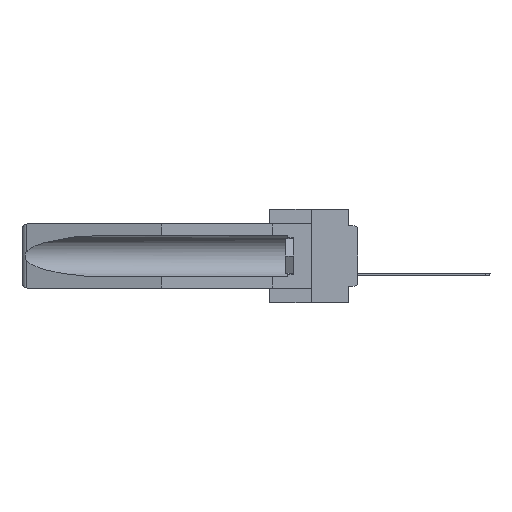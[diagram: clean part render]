
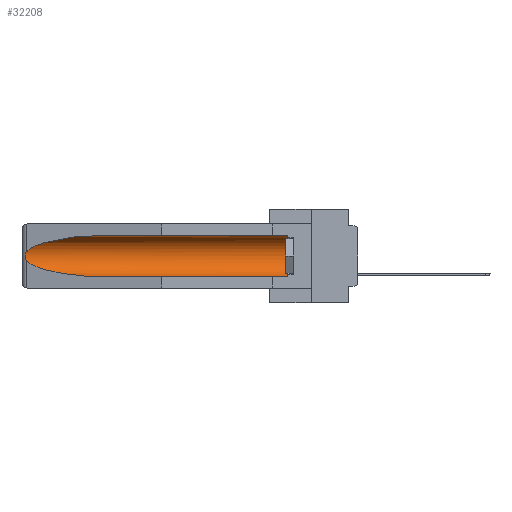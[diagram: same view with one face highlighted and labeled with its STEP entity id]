
A CAD part, left-side view. The second image highlights one B-rep face of the part: STEP entity #32208.
In plain terms, the highlighted cylindrical face has radius 2.857 mm (diameter 5.715 mm), a partial arc.
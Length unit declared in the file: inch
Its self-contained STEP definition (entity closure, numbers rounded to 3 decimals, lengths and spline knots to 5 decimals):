
#1415 = LINE ( 'NONE', #34284, #30825 ) ;
#1539 = VERTEX_POINT ( 'NONE', #34513 ) ;
#1839 = ORIENTED_EDGE ( 'NONE', *, *, #25517, .T. ) ;
#2169 = ORIENTED_EDGE ( 'NONE', *, *, #26123, .T. ) ;
#2974 = ORIENTED_EDGE ( 'NONE', *, *, #4304, .T. ) ;
#4304 = EDGE_CURVE ( 'NONE', #13439, #25281, #10258, .T. ) ;
#6087 = DIRECTION ( 'NONE',  ( 0., 0., 1. ) ) ;
#6419 = DIRECTION ( 'NONE',  ( 0., 1., 0. ) ) ;
#6476 = EDGE_LOOP ( 'NONE', ( #1839, #2169, #2974, #25697, #29636, #35950 ) ) ;
#7685 = CARTESIAN_POINT ( 'NONE',  ( 0.2675, 1.53308, -0.17534 ) ) ;
#7814 = CARTESIAN_POINT ( 'NONE',  ( 0.26655, 1.53094, -0.18657 ) ) ;
#7979 = EDGE_CURVE ( 'NONE', #1539, #15425, #1415, .T. ) ;
#8011 = CARTESIAN_POINT ( 'NONE',  ( 0.21114, 1.30732, -0.059 ) ) ;
#8209 = B_SPLINE_CURVE_WITH_KNOTS ( 'NONE', 3,
 ( #33519, #21757, #10420, #19123, #33636, #7685, #10538, #7814, #36363, #19242 ),
 .UNSPECIFIED., .F., .F.,
 ( 4, 2, 2, 2, 4 ),
 ( 0., 0.00029, 0.00058, 0.00087, 0.00117 ),
 .UNSPECIFIED. ) ;
#8282 = CARTESIAN_POINT ( 'NONE',  ( 0.155, 1.07973, -0.059 ) ) ;
#9060 = DIRECTION ( 'NONE',  ( 0., 1., 0. ) ) ;
#9190 = CARTESIAN_POINT ( 'NONE',  ( 0.155, 0.126, -0.1715 ) ) ;
#9321 = CARTESIAN_POINT ( 'NONE',  ( 0.26537, 1.52718, -0.19328 ) ) ;
#9577 = VECTOR ( 'NONE', #21256, 39.37008 ) ;
#10258 =( BOUNDED_CURVE ( )  B_SPLINE_CURVE ( 3, ( #12461, #18230, #12601, #12848 ),
 .UNSPECIFIED., .F., .F. ) 
 B_SPLINE_CURVE_WITH_KNOTS ( ( 4, 4 ),
 ( 0.1948, 1.5708 ),
 .UNSPECIFIED. ) 
 CURVE ( )  GEOMETRIC_REPRESENTATION_ITEM ( )  RATIONAL_B_SPLINE_CURVE ( ( 1., 0.848, 0.848, 1. ) ) 
 REPRESENTATION_ITEM ( '' )  );
#10420 = CARTESIAN_POINT ( 'NONE',  ( 0.26654, 1.53092, -0.15636 ) ) ;
#10538 = CARTESIAN_POINT ( 'NONE',  ( 0.2673, 1.53269, -0.17917 ) ) ;
#12461 = CARTESIAN_POINT ( 'NONE',  ( 0.26537, 1.52718, -0.19328 ) ) ;
#12601 = CARTESIAN_POINT ( 'NONE',  ( 0.21114, 1.30732, -0.284 ) ) ;
#12848 = CARTESIAN_POINT ( 'NONE',  ( 0.155, 1.07973, -0.284 ) ) ;
#13439 = VERTEX_POINT ( 'NONE', #9321 ) ;
#13619 =( BOUNDED_CURVE ( )  B_SPLINE_CURVE ( 3, ( #19319, #8011, #13673, #33702 ),
 .UNSPECIFIED., .F., .F. ) 
 B_SPLINE_CURVE_WITH_KNOTS ( ( 4, 4 ),
 ( 4.71239, 6.08839 ),
 .UNSPECIFIED. ) 
 CURVE ( )  GEOMETRIC_REPRESENTATION_ITEM ( )  RATIONAL_B_SPLINE_CURVE ( ( 1., 0.848, 0.848, 1. ) ) 
 REPRESENTATION_ITEM ( '' )  );
#13673 = CARTESIAN_POINT ( 'NONE',  ( 0.25451, 1.48313, -0.09465 ) ) ;
#15425 = VERTEX_POINT ( 'NONE', #8282 ) ;
#15603 = CARTESIAN_POINT ( 'NONE',  ( 0.155, -0.30754, -0.284 ) ) ;
#16137 = VERTEX_POINT ( 'NONE', #36723 ) ;
#17219 = VERTEX_POINT ( 'NONE', #23755 ) ;
#17978 = CARTESIAN_POINT ( 'NONE',  ( 0.155, -0.30754, -0.1715 ) ) ;
#18230 = CARTESIAN_POINT ( 'NONE',  ( 0.25451, 1.48313, -0.24835 ) ) ;
#19123 = CARTESIAN_POINT ( 'NONE',  ( 0.2673, 1.5327, -0.16383 ) ) ;
#19242 = CARTESIAN_POINT ( 'NONE',  ( 0.26537, 1.52718, -0.19328 ) ) ;
#19319 = CARTESIAN_POINT ( 'NONE',  ( 0.155, 1.07973, -0.059 ) ) ;
#20287 = AXIS2_PLACEMENT_3D ( 'NONE', #17978, #6419, #23370 ) ;
#21256 = DIRECTION ( 'NONE',  ( 0., 1., 0. ) ) ;
#21757 = CARTESIAN_POINT ( 'NONE',  ( 0.26597, 1.52961, -0.15275 ) ) ;
#22207 = AXIS2_PLACEMENT_3D ( 'NONE', #9190, #26009, #6087 ) ;
#23370 = DIRECTION ( 'NONE',  ( 0., 0., 1. ) ) ;
#23394 = LINE ( 'NONE', #15603, #9577 ) ;
#23755 = CARTESIAN_POINT ( 'NONE',  ( 0.26537, 1.52718, -0.14972 ) ) ;
#25281 = VERTEX_POINT ( 'NONE', #32586 ) ;
#25517 = EDGE_CURVE ( 'NONE', #15425, #17219, #13619, .T. ) ;
#25697 = ORIENTED_EDGE ( 'NONE', *, *, #27716, .F. ) ;
#25784 = EDGE_CURVE ( 'NONE', #16137, #1539, #33454, .T. ) ;
#26009 = DIRECTION ( 'NONE',  ( 0., -1., 0. ) ) ;
#26123 = EDGE_CURVE ( 'NONE', #17219, #13439, #8209, .T. ) ;
#27716 = EDGE_CURVE ( 'NONE', #16137, #25281, #23394, .T. ) ;
#29636 = ORIENTED_EDGE ( 'NONE', *, *, #25784, .T. ) ;
#30825 = VECTOR ( 'NONE', #9060, 39.37008 ) ;
#30958 = CYLINDRICAL_SURFACE ( 'NONE', #20287, 0.1125 ) ;
#32208 = ADVANCED_FACE ( 'NONE', ( #32749 ), #30958, .F. ) ;
#32586 = CARTESIAN_POINT ( 'NONE',  ( 0.155, 1.07973, -0.284 ) ) ;
#32749 = FACE_OUTER_BOUND ( 'NONE', #6476, .T. ) ;
#33454 = CIRCLE ( 'NONE', #22207, 0.1125 ) ;
#33519 = CARTESIAN_POINT ( 'NONE',  ( 0.26537, 1.52718, -0.14972 ) ) ;
#33636 = CARTESIAN_POINT ( 'NONE',  ( 0.2675, 1.53308, -0.16763 ) ) ;
#33702 = CARTESIAN_POINT ( 'NONE',  ( 0.26537, 1.52718, -0.14972 ) ) ;
#34284 = CARTESIAN_POINT ( 'NONE',  ( 0.155, -0.30754, -0.059 ) ) ;
#34513 = CARTESIAN_POINT ( 'NONE',  ( 0.155, 0.126, -0.059 ) ) ;
#35950 = ORIENTED_EDGE ( 'NONE', *, *, #7979, .T. ) ;
#36363 = CARTESIAN_POINT ( 'NONE',  ( 0.26597, 1.5296, -0.19026 ) ) ;
#36723 = CARTESIAN_POINT ( 'NONE',  ( 0.155, 0.126, -0.284 ) ) ;
